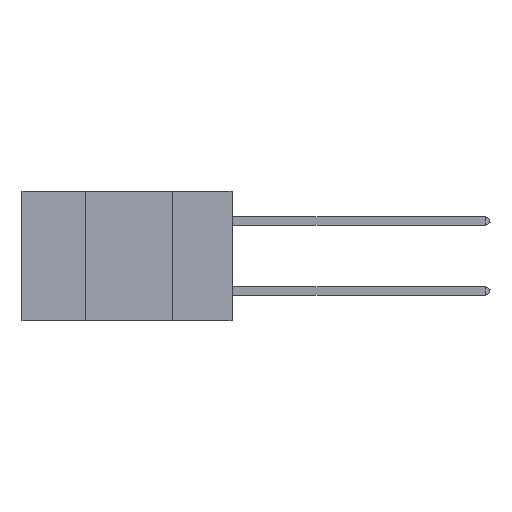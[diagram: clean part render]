
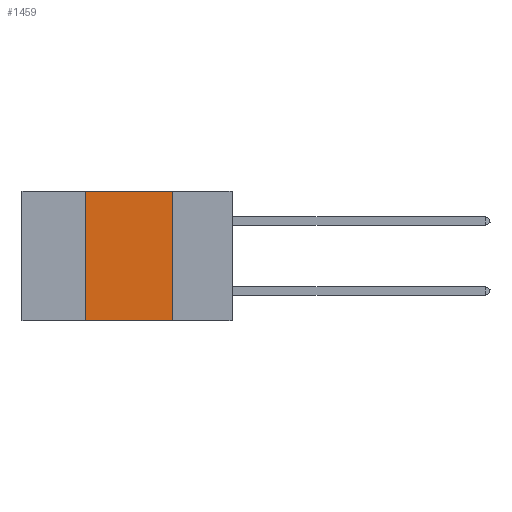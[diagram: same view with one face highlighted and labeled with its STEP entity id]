
A CAD part, left-side view. The second image highlights one B-rep face of the part: STEP entity #1459.
In plain terms, the highlighted planar face has unit normal (-1, 0, 0).
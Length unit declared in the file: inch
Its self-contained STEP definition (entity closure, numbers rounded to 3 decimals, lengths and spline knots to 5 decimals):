
#291 = VECTOR ( 'NONE', #6559, 39.37008 ) ;
#1417 = EDGE_CURVE ( 'NONE', #17593, #7558, #4888, .T. ) ;
#1459 = ADVANCED_FACE ( 'NONE', ( #3738 ), #2810, .F. ) ;
#2575 = VECTOR ( 'NONE', #8247, 39.37008 ) ;
#2810 = PLANE ( 'NONE',  #18369 ) ;
#3738 = FACE_OUTER_BOUND ( 'NONE', #11831, .T. ) ;
#3857 = CARTESIAN_POINT ( 'NONE',  ( 0., 0.17, 0. ) ) ;
#4819 = DIRECTION ( 'NONE',  ( 0., 0., -1. ) ) ;
#4888 = LINE ( 'NONE', #21444, #2575 ) ;
#6559 = DIRECTION ( 'NONE',  ( 0., 0., 1. ) ) ;
#7102 = CARTESIAN_POINT ( 'NONE',  ( 0., 0.6, 0. ) ) ;
#7558 = VERTEX_POINT ( 'NONE', #15549 ) ;
#8247 = DIRECTION ( 'NONE',  ( 0., 0., -1. ) ) ;
#8302 = VERTEX_POINT ( 'NONE', #19875 ) ;
#9264 = LINE ( 'NONE', #22105, #291 ) ;
#9447 = EDGE_CURVE ( 'NONE', #10813, #8302, #9264, .T. ) ;
#10215 = DIRECTION ( 'NONE',  ( 1., 0., 0. ) ) ;
#10813 = VERTEX_POINT ( 'NONE', #13737 ) ;
#10977 = LINE ( 'NONE', #16527, #12165 ) ;
#11729 = VECTOR ( 'NONE', #14893, 39.37008 ) ;
#11831 = EDGE_LOOP ( 'NONE', ( #18061, #16699, #21844, #16034 ) ) ;
#12165 = VECTOR ( 'NONE', #21901, 39.37008 ) ;
#13737 = CARTESIAN_POINT ( 'NONE',  ( 0., 0.42, -0.37 ) ) ;
#14183 = CARTESIAN_POINT ( 'NONE',  ( 0., 0.6, 0. ) ) ;
#14893 = DIRECTION ( 'NONE',  ( 0., -1., 0. ) ) ;
#15549 = CARTESIAN_POINT ( 'NONE',  ( 0., 0.17, -0.37 ) ) ;
#16034 = ORIENTED_EDGE ( 'NONE', *, *, #23414, .T. ) ;
#16527 = CARTESIAN_POINT ( 'NONE',  ( 0., 0.6, -0.37 ) ) ;
#16699 = ORIENTED_EDGE ( 'NONE', *, *, #20380, .F. ) ;
#17593 = VERTEX_POINT ( 'NONE', #3857 ) ;
#18061 = ORIENTED_EDGE ( 'NONE', *, *, #1417, .F. ) ;
#18369 = AXIS2_PLACEMENT_3D ( 'NONE', #14183, #10215, #4819 ) ;
#19875 = CARTESIAN_POINT ( 'NONE',  ( 0., 0.42, 0. ) ) ;
#20380 = EDGE_CURVE ( 'NONE', #8302, #17593, #22909, .T. ) ;
#21444 = CARTESIAN_POINT ( 'NONE',  ( 0., 0.17, 0. ) ) ;
#21844 = ORIENTED_EDGE ( 'NONE', *, *, #9447, .F. ) ;
#21901 = DIRECTION ( 'NONE',  ( 0., -1., 0. ) ) ;
#22105 = CARTESIAN_POINT ( 'NONE',  ( 0., 0.42, 0. ) ) ;
#22909 = LINE ( 'NONE', #7102, #11729 ) ;
#23414 = EDGE_CURVE ( 'NONE', #10813, #7558, #10977, .T. ) ;
